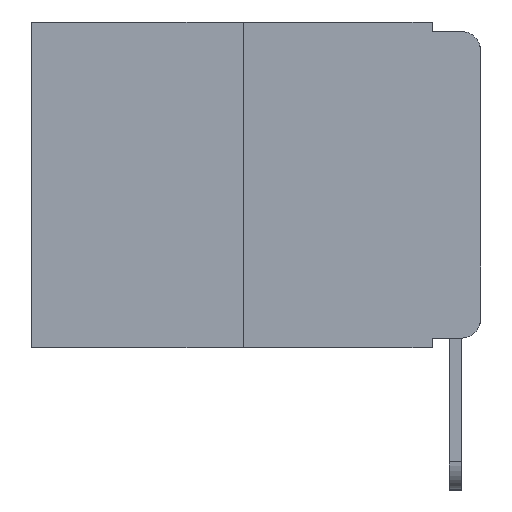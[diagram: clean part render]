
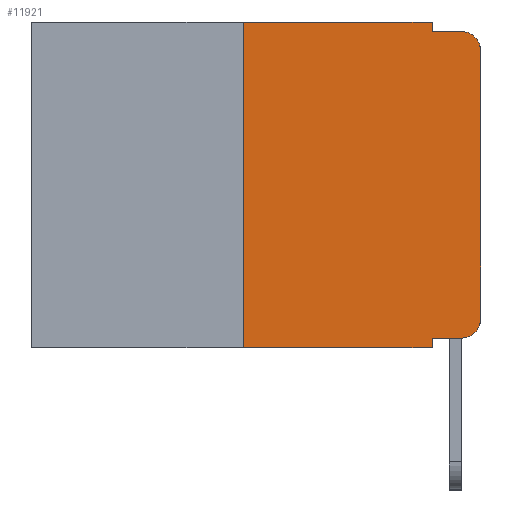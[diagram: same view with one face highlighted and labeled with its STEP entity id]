
A CAD part, left-side view. The second image highlights one B-rep face of the part: STEP entity #11921.
In plain terms, the highlighted planar face has unit normal (-1, 0, 0).
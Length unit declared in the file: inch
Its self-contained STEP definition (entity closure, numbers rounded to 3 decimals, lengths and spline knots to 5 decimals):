
#286 = DIRECTION ( 'NONE',  ( 1., 0., 0. ) ) ;
#349 = ORIENTED_EDGE ( 'NONE', *, *, #664, .T. ) ;
#456 = VERTEX_POINT ( 'NONE', #627 ) ;
#614 = EDGE_CURVE ( 'NONE', #997, #9387, #9763, .T. ) ;
#627 = CARTESIAN_POINT ( 'NONE',  ( 0., 0.051, 0. ) ) ;
#646 = CARTESIAN_POINT ( 'NONE',  ( 0., 0.02, -0.313 ) ) ;
#664 = EDGE_CURVE ( 'NONE', #9622, #10255, #7705, .T. ) ;
#680 = CARTESIAN_POINT ( 'NONE',  ( 0., 0.473, 0. ) ) ;
#739 = CARTESIAN_POINT ( 'NONE',  ( 0., 0.051, -0.333 ) ) ;
#997 = VERTEX_POINT ( 'NONE', #1084 ) ;
#1084 = CARTESIAN_POINT ( 'NONE',  ( 0., 0.25, -0.343 ) ) ;
#1116 = CIRCLE ( 'NONE', #6076, 0.02 ) ;
#1431 = EDGE_CURVE ( 'NONE', #2709, #9622, #1116, .T. ) ;
#1443 = DIRECTION ( 'NONE',  ( 0., 0., 1. ) ) ;
#1453 = LINE ( 'NONE', #9126, #11327 ) ;
#1462 = ORIENTED_EDGE ( 'NONE', *, *, #3034, .F. ) ;
#2502 = VECTOR ( 'NONE', #3992, 39.37008 ) ;
#2506 = EDGE_CURVE ( 'NONE', #3841, #2709, #11062, .T. ) ;
#2653 = VECTOR ( 'NONE', #1443, 39.37008 ) ;
#2709 = VERTEX_POINT ( 'NONE', #6912 ) ;
#2884 = EDGE_CURVE ( 'NONE', #10255, #6842, #7808, .T. ) ;
#3034 = EDGE_CURVE ( 'NONE', #5457, #6842, #1453, .T. ) ;
#3403 = CARTESIAN_POINT ( 'NONE',  ( 0., 0.25, 0. ) ) ;
#3434 = VECTOR ( 'NONE', #12142, 39.37008 ) ;
#3596 = VECTOR ( 'NONE', #9365, 39.37008 ) ;
#3601 = EDGE_CURVE ( 'NONE', #456, #5457, #5568, .T. ) ;
#3841 = VERTEX_POINT ( 'NONE', #739 ) ;
#3992 = DIRECTION ( 'NONE',  ( 0., -1., 0. ) ) ;
#4056 = AXIS2_PLACEMENT_3D ( 'NONE', #11543, #11574, #8957 ) ;
#4077 = VECTOR ( 'NONE', #4314, 39.37008 ) ;
#4250 = CARTESIAN_POINT ( 'NONE',  ( 0., 0.051, -0.01 ) ) ;
#4314 = DIRECTION ( 'NONE',  ( 0., 0., -1. ) ) ;
#4385 = DIRECTION ( 'NONE',  ( 0., 0., 1. ) ) ;
#4395 = LINE ( 'NONE', #11703, #4077 ) ;
#4559 = PLANE ( 'NONE',  #11146 ) ;
#5276 = VECTOR ( 'NONE', #8094, 39.37008 ) ;
#5343 = EDGE_CURVE ( 'NONE', #9314, #456, #6038, .T. ) ;
#5381 = ORIENTED_EDGE ( 'NONE', *, *, #2506, .T. ) ;
#5457 = VERTEX_POINT ( 'NONE', #4250 ) ;
#5568 = LINE ( 'NONE', #9597, #5276 ) ;
#5658 = CARTESIAN_POINT ( 'NONE',  ( 0., 0., 0. ) ) ;
#5676 = ORIENTED_EDGE ( 'NONE', *, *, #614, .T. ) ;
#6038 = LINE ( 'NONE', #680, #3434 ) ;
#6076 = AXIS2_PLACEMENT_3D ( 'NONE', #646, #10275, #7984 ) ;
#6249 = ORIENTED_EDGE ( 'NONE', *, *, #7082, .F. ) ;
#6451 = CARTESIAN_POINT ( 'NONE',  ( 0., 0.473, -0.343 ) ) ;
#6548 = ORIENTED_EDGE ( 'NONE', *, *, #5343, .F. ) ;
#6583 = VECTOR ( 'NONE', #4385, 39.37008 ) ;
#6667 = CARTESIAN_POINT ( 'NONE',  ( 0., 0.25, 0. ) ) ;
#6842 = VERTEX_POINT ( 'NONE', #9180 ) ;
#6912 = CARTESIAN_POINT ( 'NONE',  ( 0., 0.02, -0.333 ) ) ;
#7082 = EDGE_CURVE ( 'NONE', #997, #9314, #8941, .T. ) ;
#7342 = DIRECTION ( 'NONE',  ( 0., 0., -1. ) ) ;
#7583 = CARTESIAN_POINT ( 'NONE',  ( 0., 0., -0.03 ) ) ;
#7705 = LINE ( 'NONE', #5658, #2653 ) ;
#7748 = ORIENTED_EDGE ( 'NONE', *, *, #1431, .T. ) ;
#7808 = CIRCLE ( 'NONE', #4056, 0.02 ) ;
#7984 = DIRECTION ( 'NONE',  ( 0., 0., -1. ) ) ;
#8011 = ORIENTED_EDGE ( 'NONE', *, *, #12391, .F. ) ;
#8094 = DIRECTION ( 'NONE',  ( 0., 0., -1. ) ) ;
#8566 = CARTESIAN_POINT ( 'NONE',  ( 0., 0.051, -0.343 ) ) ;
#8941 = LINE ( 'NONE', #3403, #6583 ) ;
#8957 = DIRECTION ( 'NONE',  ( 0., 0., -1. ) ) ;
#9126 = CARTESIAN_POINT ( 'NONE',  ( 0., 0.051, -0.01 ) ) ;
#9129 = CARTESIAN_POINT ( 'NONE',  ( 0., 0.473, 0. ) ) ;
#9180 = CARTESIAN_POINT ( 'NONE',  ( 0., 0.02, -0.01 ) ) ;
#9314 = VERTEX_POINT ( 'NONE', #6667 ) ;
#9365 = DIRECTION ( 'NONE',  ( 0., -1., 0. ) ) ;
#9387 = VERTEX_POINT ( 'NONE', #8566 ) ;
#9597 = CARTESIAN_POINT ( 'NONE',  ( 0., 0.051, 0. ) ) ;
#9622 = VERTEX_POINT ( 'NONE', #10893 ) ;
#9666 = ORIENTED_EDGE ( 'NONE', *, *, #2884, .T. ) ;
#9763 = LINE ( 'NONE', #6451, #2502 ) ;
#9943 = CARTESIAN_POINT ( 'NONE',  ( 0., 0.051, -0.333 ) ) ;
#9968 = ORIENTED_EDGE ( 'NONE', *, *, #3601, .F. ) ;
#10255 = VERTEX_POINT ( 'NONE', #7583 ) ;
#10275 = DIRECTION ( 'NONE',  ( -1., 0., 0. ) ) ;
#10893 = CARTESIAN_POINT ( 'NONE',  ( 0., 0., -0.313 ) ) ;
#11062 = LINE ( 'NONE', #9943, #3596 ) ;
#11067 = DIRECTION ( 'NONE',  ( 0., -1., 0. ) ) ;
#11146 = AXIS2_PLACEMENT_3D ( 'NONE', #9129, #286, #7342 ) ;
#11327 = VECTOR ( 'NONE', #11067, 39.37008 ) ;
#11543 = CARTESIAN_POINT ( 'NONE',  ( 0., 0.02, -0.03 ) ) ;
#11574 = DIRECTION ( 'NONE',  ( -1., 0., 0. ) ) ;
#11703 = CARTESIAN_POINT ( 'NONE',  ( 0., 0.051, 0. ) ) ;
#11921 = ADVANCED_FACE ( 'NONE', ( #12310 ), #4559, .F. ) ;
#11936 = EDGE_LOOP ( 'NONE', ( #349, #9666, #1462, #9968, #6548, #6249, #5676, #8011, #5381, #7748 ) ) ;
#12142 = DIRECTION ( 'NONE',  ( 0., -1., 0. ) ) ;
#12310 = FACE_OUTER_BOUND ( 'NONE', #11936, .T. ) ;
#12391 = EDGE_CURVE ( 'NONE', #3841, #9387, #4395, .T. ) ;
